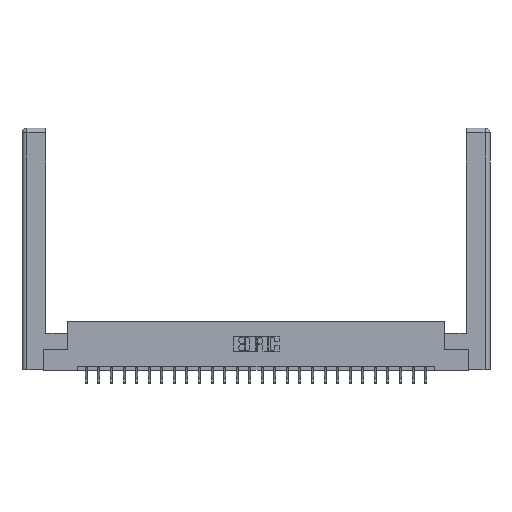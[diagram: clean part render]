
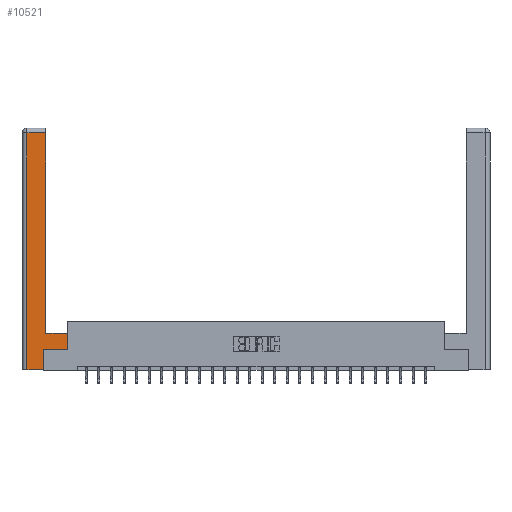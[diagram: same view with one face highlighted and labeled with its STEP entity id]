
A CAD part, top view. The second image highlights one B-rep face of the part: STEP entity #10521.
In plain terms, the highlighted planar face has unit normal (0, 0, 1).
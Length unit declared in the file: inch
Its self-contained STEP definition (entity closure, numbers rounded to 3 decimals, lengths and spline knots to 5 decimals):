
#282 = VERTEX_POINT ( 'NONE', #15358 ) ;
#465 = ORIENTED_EDGE ( 'NONE', *, *, #12134, .T. ) ;
#1525 = EDGE_CURVE ( 'NONE', #7338, #15795, #1878, .T. ) ;
#1878 = LINE ( 'NONE', #17280, #19479 ) ;
#2878 = DIRECTION ( 'NONE',  ( 0., -1., 0. ) ) ;
#3092 = EDGE_CURVE ( 'NONE', #21056, #10211, #22605, .T. ) ;
#4166 = VECTOR ( 'NONE', #7037, 39.37008 ) ;
#4723 = ORIENTED_EDGE ( 'NONE', *, *, #11547, .T. ) ;
#4814 = LINE ( 'NONE', #11827, #5784 ) ;
#5010 = CARTESIAN_POINT ( 'NONE',  ( 0.295, 0.45, 0. ) ) ;
#5077 = CARTESIAN_POINT ( 'NONE',  ( 0.565, 0.45, 0. ) ) ;
#5784 = VECTOR ( 'NONE', #8176, 39.37008 ) ;
#5817 = LINE ( 'NONE', #6172, #24238 ) ;
#6161 = DIRECTION ( 'NONE',  ( 0., 1., 0. ) ) ;
#6172 = CARTESIAN_POINT ( 'NONE',  ( 0.265, 0., 0. ) ) ;
#6189 = ORIENTED_EDGE ( 'NONE', *, *, #18936, .T. ) ;
#6290 = DIRECTION ( 'NONE',  ( -1., 0., 0. ) ) ;
#6839 = VECTOR ( 'NONE', #6161, 39.37008 ) ;
#7037 = DIRECTION ( 'NONE',  ( 0., 1., 0. ) ) ;
#7172 = CARTESIAN_POINT ( 'NONE',  ( 0.295, 3., 0. ) ) ;
#7288 = VECTOR ( 'NONE', #22295, 39.37008 ) ;
#7338 = VERTEX_POINT ( 'NONE', #15219 ) ;
#7829 = VERTEX_POINT ( 'NONE', #22091 ) ;
#8176 = DIRECTION ( 'NONE',  ( -1., 0., 0. ) ) ;
#8958 = EDGE_LOOP ( 'NONE', ( #6189, #4723, #16085, #11091, #16480, #23557, #16608, #465 ) ) ;
#9196 = CARTESIAN_POINT ( 'NONE',  ( 0., 0., 0. ) ) ;
#10211 = VERTEX_POINT ( 'NONE', #26073 ) ;
#10478 = CARTESIAN_POINT ( 'NONE',  ( 0.0615, 0., 0. ) ) ;
#10521 = ADVANCED_FACE ( 'NONE', ( #20582 ), #17249, .F. ) ;
#10569 = CARTESIAN_POINT ( 'NONE',  ( 0.295, 0.45, 0. ) ) ;
#10643 = DIRECTION ( 'NONE',  ( 0., 1., 0. ) ) ;
#11091 = ORIENTED_EDGE ( 'NONE', *, *, #20287, .T. ) ;
#11420 = DIRECTION ( 'NONE',  ( 0., 0., -1. ) ) ;
#11547 = EDGE_CURVE ( 'NONE', #22568, #7338, #4814, .T. ) ;
#11827 = CARTESIAN_POINT ( 'NONE',  ( 0.0615, 2.94, 0. ) ) ;
#12134 = EDGE_CURVE ( 'NONE', #7829, #14373, #23617, .T. ) ;
#14373 = VERTEX_POINT ( 'NONE', #5010 ) ;
#14738 = EDGE_CURVE ( 'NONE', #282, #21056, #19192, .T. ) ;
#15219 = CARTESIAN_POINT ( 'NONE',  ( 0.0615, 2.94, 0. ) ) ;
#15358 = CARTESIAN_POINT ( 'NONE',  ( 0.265, 0., 0. ) ) ;
#15795 = VERTEX_POINT ( 'NONE', #10478 ) ;
#16085 = ORIENTED_EDGE ( 'NONE', *, *, #1525, .T. ) ;
#16480 = ORIENTED_EDGE ( 'NONE', *, *, #14738, .T. ) ;
#16608 = ORIENTED_EDGE ( 'NONE', *, *, #17151, .T. ) ;
#17151 = EDGE_CURVE ( 'NONE', #10211, #7829, #22585, .T. ) ;
#17249 = PLANE ( 'NONE',  #19963 ) ;
#17280 = CARTESIAN_POINT ( 'NONE',  ( 0.0615, 0., 0. ) ) ;
#18310 = CARTESIAN_POINT ( 'NONE',  ( 0.565, 0.245, 0. ) ) ;
#18936 = EDGE_CURVE ( 'NONE', #14373, #22568, #25656, .T. ) ;
#19192 = LINE ( 'NONE', #19282, #4166 ) ;
#19282 = CARTESIAN_POINT ( 'NONE',  ( 0.265, 0.245, 0. ) ) ;
#19479 = VECTOR ( 'NONE', #2878, 39.37008 ) ;
#19963 = AXIS2_PLACEMENT_3D ( 'NONE', #9196, #11420, #25658 ) ;
#20287 = EDGE_CURVE ( 'NONE', #15795, #282, #5817, .T. ) ;
#20582 = FACE_OUTER_BOUND ( 'NONE', #8958, .T. ) ;
#20720 = VECTOR ( 'NONE', #10643, 39.37008 ) ;
#21056 = VERTEX_POINT ( 'NONE', #25437 ) ;
#22091 = CARTESIAN_POINT ( 'NONE',  ( 0.565, 0.45, 0. ) ) ;
#22295 = DIRECTION ( 'NONE',  ( 1., 0., 0. ) ) ;
#22315 = DIRECTION ( 'NONE',  ( 1., 0., 0. ) ) ;
#22356 = VECTOR ( 'NONE', #6290, 39.37008 ) ;
#22474 = CARTESIAN_POINT ( 'NONE',  ( 0.295, 2.94, 0. ) ) ;
#22568 = VERTEX_POINT ( 'NONE', #22474 ) ;
#22585 = LINE ( 'NONE', #5077, #20720 ) ;
#22605 = LINE ( 'NONE', #18310, #7288 ) ;
#23557 = ORIENTED_EDGE ( 'NONE', *, *, #3092, .T. ) ;
#23617 = LINE ( 'NONE', #10569, #22356 ) ;
#24238 = VECTOR ( 'NONE', #22315, 39.37008 ) ;
#25437 = CARTESIAN_POINT ( 'NONE',  ( 0.265, 0.245, 0. ) ) ;
#25656 = LINE ( 'NONE', #7172, #6839 ) ;
#25658 = DIRECTION ( 'NONE',  ( -1., 0., 0. ) ) ;
#26073 = CARTESIAN_POINT ( 'NONE',  ( 0.565, 0.245, 0. ) ) ;
